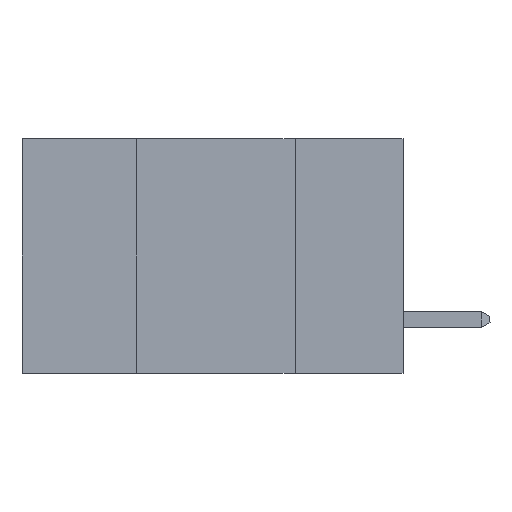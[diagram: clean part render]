
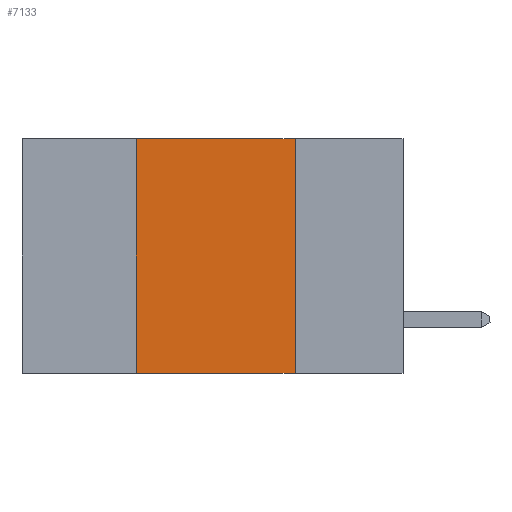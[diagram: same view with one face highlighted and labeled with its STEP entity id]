
A CAD part, left-side view. The second image highlights one B-rep face of the part: STEP entity #7133.
In plain terms, the highlighted planar face has unit normal (-1, 0, 0).
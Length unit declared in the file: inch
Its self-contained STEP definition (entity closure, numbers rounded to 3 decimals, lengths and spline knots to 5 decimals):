
#28 = DIRECTION ( 'NONE',  ( 0., 0., 1. ) ) ;
#282 = ORIENTED_EDGE ( 'NONE', *, *, #14723, .F. ) ;
#632 = FACE_OUTER_BOUND ( 'NONE', #9076, .T. ) ;
#739 = EDGE_CURVE ( 'NONE', #12250, #7738, #12592, .T. ) ;
#836 = ORIENTED_EDGE ( 'NONE', *, *, #3600, .F. ) ;
#851 = ORIENTED_EDGE ( 'NONE', *, *, #11289, .F. ) ;
#894 = DIRECTION ( 'NONE',  ( 0., -1., 0. ) ) ;
#1401 = CARTESIAN_POINT ( 'NONE',  ( 0., 0.6, -0.37 ) ) ;
#2026 = CARTESIAN_POINT ( 'NONE',  ( 0., 0.42, -0.37 ) ) ;
#2147 = VECTOR ( 'NONE', #894, 39.37008 ) ;
#2643 = VERTEX_POINT ( 'NONE', #8240 ) ;
#3005 = AXIS2_PLACEMENT_3D ( 'NONE', #12169, #14719, #7017 ) ;
#3600 = EDGE_CURVE ( 'NONE', #11081, #2643, #12111, .T. ) ;
#3725 = DIRECTION ( 'NONE',  ( 0., 0., -1. ) ) ;
#4240 = DIRECTION ( 'NONE',  ( 0., -1., 0. ) ) ;
#5037 = CARTESIAN_POINT ( 'NONE',  ( 0., 0.6, 0. ) ) ;
#5849 = VECTOR ( 'NONE', #3725, 39.37008 ) ;
#6254 = CARTESIAN_POINT ( 'NONE',  ( 0., 0.42, 0. ) ) ;
#6507 = LINE ( 'NONE', #15693, #10316 ) ;
#7017 = DIRECTION ( 'NONE',  ( 0., 0., -1. ) ) ;
#7133 = ADVANCED_FACE ( 'NONE', ( #632 ), #10829, .F. ) ;
#7738 = VERTEX_POINT ( 'NONE', #9493 ) ;
#8240 = CARTESIAN_POINT ( 'NONE',  ( 0., 0.17, 0. ) ) ;
#8259 = VECTOR ( 'NONE', #4240, 39.37008 ) ;
#9076 = EDGE_LOOP ( 'NONE', ( #282, #836, #851, #10209 ) ) ;
#9493 = CARTESIAN_POINT ( 'NONE',  ( 0., 0.17, -0.37 ) ) ;
#10209 = ORIENTED_EDGE ( 'NONE', *, *, #739, .T. ) ;
#10316 = VECTOR ( 'NONE', #28, 39.37008 ) ;
#10829 = PLANE ( 'NONE',  #3005 ) ;
#11081 = VERTEX_POINT ( 'NONE', #6254 ) ;
#11289 = EDGE_CURVE ( 'NONE', #12250, #11081, #6507, .T. ) ;
#11563 = CARTESIAN_POINT ( 'NONE',  ( 0., 0.17, 0. ) ) ;
#12111 = LINE ( 'NONE', #5037, #8259 ) ;
#12169 = CARTESIAN_POINT ( 'NONE',  ( 0., 0.6, 0. ) ) ;
#12250 = VERTEX_POINT ( 'NONE', #2026 ) ;
#12592 = LINE ( 'NONE', #1401, #2147 ) ;
#14719 = DIRECTION ( 'NONE',  ( 1., 0., 0. ) ) ;
#14723 = EDGE_CURVE ( 'NONE', #2643, #7738, #16140, .T. ) ;
#15693 = CARTESIAN_POINT ( 'NONE',  ( 0., 0.42, 0. ) ) ;
#16140 = LINE ( 'NONE', #11563, #5849 ) ;
